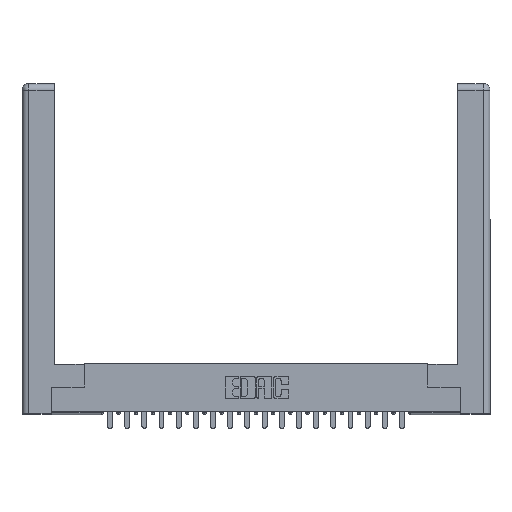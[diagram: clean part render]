
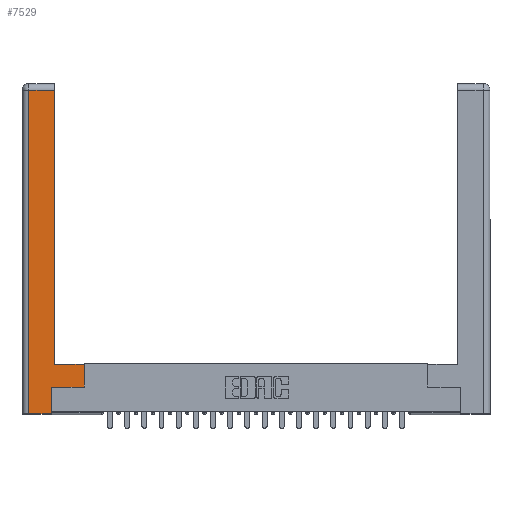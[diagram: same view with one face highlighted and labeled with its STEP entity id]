
A CAD part, top view. The second image highlights one B-rep face of the part: STEP entity #7529.
In plain terms, the highlighted planar face has unit normal (0, 0, 1).
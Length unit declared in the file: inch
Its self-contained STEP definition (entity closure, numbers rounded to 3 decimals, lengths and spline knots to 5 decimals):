
#143 = VECTOR ( 'NONE', #13885, 39.37008 ) ;
#879 = ORIENTED_EDGE ( 'NONE', *, *, #15511, .T. ) ;
#1067 = PLANE ( 'NONE',  #22903 ) ;
#1128 = DIRECTION ( 'NONE',  ( 0., 1., 0. ) ) ;
#1157 = EDGE_LOOP ( 'NONE', ( #13343, #17973, #8682, #21069, #879, #20696, #9284, #7575 ) ) ;
#1363 = CARTESIAN_POINT ( 'NONE',  ( 0.565, 0.45, 0. ) ) ;
#2350 = CARTESIAN_POINT ( 'NONE',  ( 0.295, 0.45, 0. ) ) ;
#2670 = CARTESIAN_POINT ( 'NONE',  ( 0.295, 3., 0. ) ) ;
#2792 = CARTESIAN_POINT ( 'NONE',  ( 0.295, 2.94, 0. ) ) ;
#2843 = DIRECTION ( 'NONE',  ( -1., 0., 0. ) ) ;
#3584 = CARTESIAN_POINT ( 'NONE',  ( 0.265, 0., 0. ) ) ;
#4211 = DIRECTION ( 'NONE',  ( -1., 0., 0. ) ) ;
#4273 = CARTESIAN_POINT ( 'NONE',  ( 0.265, 0.245, 0. ) ) ;
#4869 = CARTESIAN_POINT ( 'NONE',  ( 0.565, 0.245, 0. ) ) ;
#4967 = LINE ( 'NONE', #23302, #143 ) ;
#6254 = VECTOR ( 'NONE', #4211, 39.37008 ) ;
#6264 = VERTEX_POINT ( 'NONE', #19787 ) ;
#6449 = DIRECTION ( 'NONE',  ( -1., 0., 0. ) ) ;
#7226 = LINE ( 'NONE', #1363, #18058 ) ;
#7310 = VECTOR ( 'NONE', #9652, 39.37008 ) ;
#7529 = ADVANCED_FACE ( 'NONE', ( #12626 ), #1067, .F. ) ;
#7575 = ORIENTED_EDGE ( 'NONE', *, *, #19674, .T. ) ;
#8301 = VECTOR ( 'NONE', #19833, 39.37008 ) ;
#8682 = ORIENTED_EDGE ( 'NONE', *, *, #23699, .T. ) ;
#8691 = VECTOR ( 'NONE', #6449, 39.37008 ) ;
#8786 = DIRECTION ( 'NONE',  ( 0., 0., -1. ) ) ;
#9284 = ORIENTED_EDGE ( 'NONE', *, *, #22119, .T. ) ;
#9652 = DIRECTION ( 'NONE',  ( 1., 0., 0. ) ) ;
#11178 = VERTEX_POINT ( 'NONE', #18494 ) ;
#11944 = EDGE_CURVE ( 'NONE', #18670, #16551, #18884, .T. ) ;
#12626 = FACE_OUTER_BOUND ( 'NONE', #1157, .T. ) ;
#12928 = VERTEX_POINT ( 'NONE', #13328 ) ;
#13071 = LINE ( 'NONE', #4869, #22387 ) ;
#13328 = CARTESIAN_POINT ( 'NONE',  ( 0.265, 0., 0. ) ) ;
#13343 = ORIENTED_EDGE ( 'NONE', *, *, #13731, .T. ) ;
#13731 = EDGE_CURVE ( 'NONE', #20155, #18670, #23648, .T. ) ;
#13777 = VECTOR ( 'NONE', #16480, 39.37008 ) ;
#13829 = LINE ( 'NONE', #2350, #8691 ) ;
#13885 = DIRECTION ( 'NONE',  ( 0., 1., 0. ) ) ;
#14523 = CARTESIAN_POINT ( 'NONE',  ( 0.295, 0.45, 0. ) ) ;
#14676 = EDGE_CURVE ( 'NONE', #20544, #6264, #13071, .T. ) ;
#15511 = EDGE_CURVE ( 'NONE', #12928, #20544, #4967, .T. ) ;
#16219 = CARTESIAN_POINT ( 'NONE',  ( 0., 0., 0. ) ) ;
#16480 = DIRECTION ( 'NONE',  ( 0., -1., 0. ) ) ;
#16551 = VERTEX_POINT ( 'NONE', #18628 ) ;
#16606 = EDGE_CURVE ( 'NONE', #24075, #12928, #22674, .T. ) ;
#17736 = CARTESIAN_POINT ( 'NONE',  ( 0.0615, 2.94, 0. ) ) ;
#17817 = CARTESIAN_POINT ( 'NONE',  ( 0.0615, 0., 0. ) ) ;
#17973 = ORIENTED_EDGE ( 'NONE', *, *, #11944, .T. ) ;
#18058 = VECTOR ( 'NONE', #1128, 39.37008 ) ;
#18494 = CARTESIAN_POINT ( 'NONE',  ( 0.565, 0.45, 0. ) ) ;
#18628 = CARTESIAN_POINT ( 'NONE',  ( 0.0615, 2.94, 0. ) ) ;
#18670 = VERTEX_POINT ( 'NONE', #2792 ) ;
#18884 = LINE ( 'NONE', #17736, #6254 ) ;
#19674 = EDGE_CURVE ( 'NONE', #11178, #20155, #13829, .T. ) ;
#19787 = CARTESIAN_POINT ( 'NONE',  ( 0.565, 0.245, 0. ) ) ;
#19833 = DIRECTION ( 'NONE',  ( 0., 1., 0. ) ) ;
#20155 = VERTEX_POINT ( 'NONE', #14523 ) ;
#20544 = VERTEX_POINT ( 'NONE', #4273 ) ;
#20696 = ORIENTED_EDGE ( 'NONE', *, *, #14676, .T. ) ;
#21069 = ORIENTED_EDGE ( 'NONE', *, *, #16606, .T. ) ;
#22119 = EDGE_CURVE ( 'NONE', #6264, #11178, #7226, .T. ) ;
#22303 = CARTESIAN_POINT ( 'NONE',  ( 0.0615, 0., 0. ) ) ;
#22387 = VECTOR ( 'NONE', #22450, 39.37008 ) ;
#22450 = DIRECTION ( 'NONE',  ( 1., 0., 0. ) ) ;
#22674 = LINE ( 'NONE', #3584, #7310 ) ;
#22903 = AXIS2_PLACEMENT_3D ( 'NONE', #16219, #8786, #2843 ) ;
#23302 = CARTESIAN_POINT ( 'NONE',  ( 0.265, 0.245, 0. ) ) ;
#23648 = LINE ( 'NONE', #2670, #8301 ) ;
#23699 = EDGE_CURVE ( 'NONE', #16551, #24075, #24917, .T. ) ;
#24075 = VERTEX_POINT ( 'NONE', #17817 ) ;
#24917 = LINE ( 'NONE', #22303, #13777 ) ;
